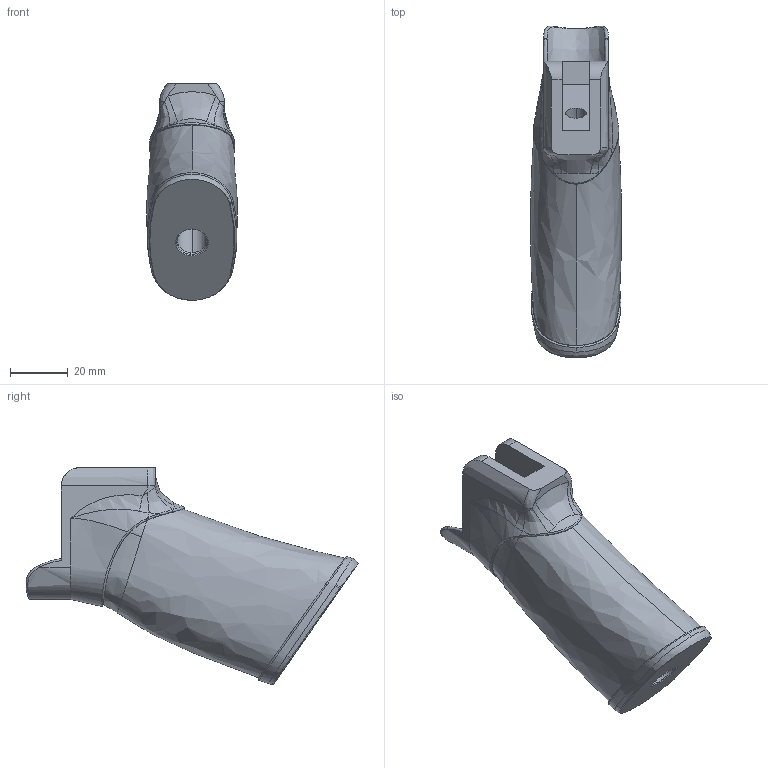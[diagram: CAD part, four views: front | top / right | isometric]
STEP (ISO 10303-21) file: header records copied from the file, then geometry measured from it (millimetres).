
FILE_DESCRIPTION (( 'STEP AP203' ), '1' );
FILE_NAME ('Grip V3.1 Milspec TR.STEP', '2022-05-14T17:18:45', ( '' ), ( '' ), 'SwSTEP 2.0', 'SolidWorks 2021', '' );
FILE_SCHEMA (( 'CONFIG_CONTROL_DESIGN' ));
Length unit declared in the file: inch
Products named in the file (1): Grip V3.1 Milspec TR
Bounding box: 31.51 x 115.21 x 75.19 mm (x, y, z)
Volume: 99398.9 mm3; surface area: 18618 mm2
Topology: 1 solids, 1 shells, 87 faces, 234 edges, 145 vertices
Faces by surface type: bspline 66, plane 13, cylinder 8
Entity records: 24874 total; most frequent: CARTESIAN_POINT 23188, ORIENTED_EDGE 456, EDGE_CURVE 228, B_SPLINE_CURVE_WITH_KNOTS 157, VERTEX_POINT 145, DIRECTION 140, EDGE_LOOP 91, FACE_OUTER_BOUND 87
